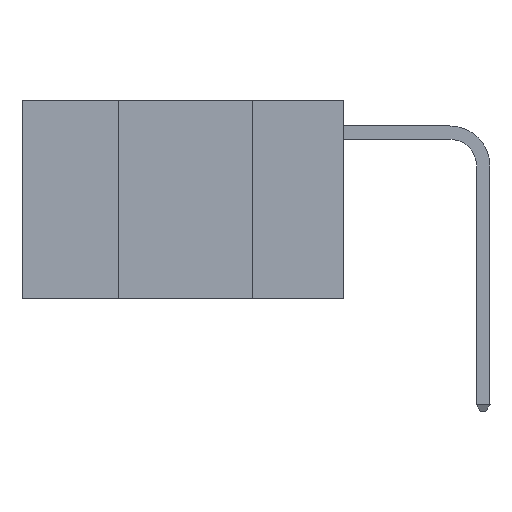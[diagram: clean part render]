
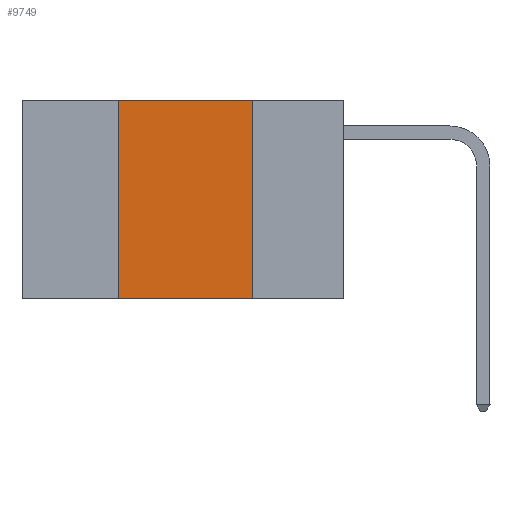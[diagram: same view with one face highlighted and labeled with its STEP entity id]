
A CAD part, left-side view. The second image highlights one B-rep face of the part: STEP entity #9749.
In plain terms, the highlighted planar face has unit normal (-1, 0, 0).
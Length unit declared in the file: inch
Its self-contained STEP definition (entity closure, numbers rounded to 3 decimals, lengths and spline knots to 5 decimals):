
#929 = VECTOR ( 'NONE', #11626, 39.37008 ) ;
#1267 = LINE ( 'NONE', #1443, #7740 ) ;
#1443 = CARTESIAN_POINT ( 'NONE',  ( 0., 0.42, 0. ) ) ;
#1586 = VERTEX_POINT ( 'NONE', #1950 ) ;
#1701 = CARTESIAN_POINT ( 'NONE',  ( 0., 0.6, 0. ) ) ;
#1803 = LINE ( 'NONE', #14245, #8255 ) ;
#1950 = CARTESIAN_POINT ( 'NONE',  ( 0., 0.42, -0.37 ) ) ;
#2043 = FACE_OUTER_BOUND ( 'NONE', #2773, .T. ) ;
#2402 = CARTESIAN_POINT ( 'NONE',  ( 0., 0.17, -0.37 ) ) ;
#2668 = CARTESIAN_POINT ( 'NONE',  ( 0., 0.17, 0. ) ) ;
#2772 = DIRECTION ( 'NONE',  ( 0., 0., 1. ) ) ;
#2773 = EDGE_LOOP ( 'NONE', ( #9849, #3690, #8189, #15799 ) ) ;
#3200 = CARTESIAN_POINT ( 'NONE',  ( 0., 0.6, 0. ) ) ;
#3690 = ORIENTED_EDGE ( 'NONE', *, *, #12860, .F. ) ;
#3993 = LINE ( 'NONE', #2668, #929 ) ;
#4339 = DIRECTION ( 'NONE',  ( 1., 0., 0. ) ) ;
#6836 = CARTESIAN_POINT ( 'NONE',  ( 0., 0.42, 0. ) ) ;
#6861 = EDGE_CURVE ( 'NONE', #1586, #6978, #1267, .T. ) ;
#6978 = VERTEX_POINT ( 'NONE', #6836 ) ;
#7740 = VECTOR ( 'NONE', #2772, 39.37008 ) ;
#7827 = LINE ( 'NONE', #3200, #10836 ) ;
#7863 = CARTESIAN_POINT ( 'NONE',  ( 0., 0.17, 0. ) ) ;
#8189 = ORIENTED_EDGE ( 'NONE', *, *, #6861, .F. ) ;
#8255 = VECTOR ( 'NONE', #15469, 39.37008 ) ;
#9749 = ADVANCED_FACE ( 'NONE', ( #2043 ), #11924, .F. ) ;
#9849 = ORIENTED_EDGE ( 'NONE', *, *, #14679, .F. ) ;
#10737 = VERTEX_POINT ( 'NONE', #2402 ) ;
#10836 = VECTOR ( 'NONE', #10898, 39.37008 ) ;
#10880 = EDGE_CURVE ( 'NONE', #1586, #10737, #1803, .T. ) ;
#10898 = DIRECTION ( 'NONE',  ( 0., -1., 0. ) ) ;
#11626 = DIRECTION ( 'NONE',  ( 0., 0., -1. ) ) ;
#11924 = PLANE ( 'NONE',  #15043 ) ;
#12622 = VERTEX_POINT ( 'NONE', #7863 ) ;
#12860 = EDGE_CURVE ( 'NONE', #6978, #12622, #7827, .T. ) ;
#13229 = DIRECTION ( 'NONE',  ( 0., 0., -1. ) ) ;
#14245 = CARTESIAN_POINT ( 'NONE',  ( 0., 0.6, -0.37 ) ) ;
#14679 = EDGE_CURVE ( 'NONE', #12622, #10737, #3993, .T. ) ;
#15043 = AXIS2_PLACEMENT_3D ( 'NONE', #1701, #4339, #13229 ) ;
#15469 = DIRECTION ( 'NONE',  ( 0., -1., 0. ) ) ;
#15799 = ORIENTED_EDGE ( 'NONE', *, *, #10880, .T. ) ;
